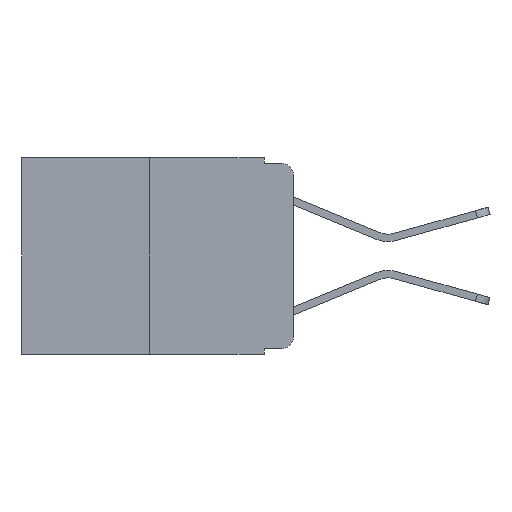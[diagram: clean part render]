
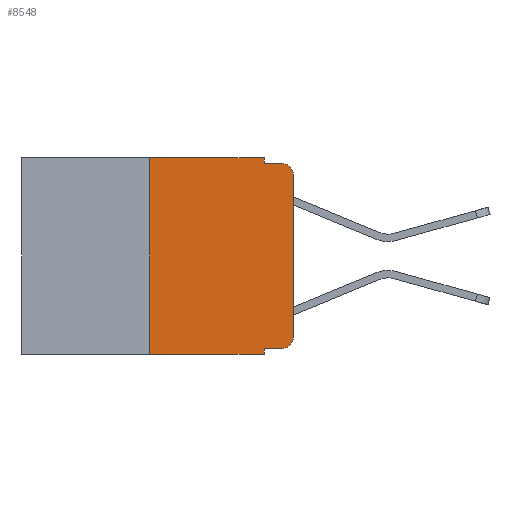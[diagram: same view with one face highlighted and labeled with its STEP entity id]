
A CAD part, left-side view. The second image highlights one B-rep face of the part: STEP entity #8548.
In plain terms, the highlighted planar face has unit normal (-1, 0, 0).
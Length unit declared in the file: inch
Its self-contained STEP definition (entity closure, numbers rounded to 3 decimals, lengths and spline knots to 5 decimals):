
#337 = ORIENTED_EDGE ( 'NONE', *, *, #23741, .T. ) ;
#712 = CARTESIAN_POINT ( 'NONE',  ( 0., 0.051, -0.01 ) ) ;
#1247 = DIRECTION ( 'NONE',  ( 0., 0., -1. ) ) ;
#1405 = LINE ( 'NONE', #23690, #12093 ) ;
#1639 = EDGE_CURVE ( 'NONE', #9684, #12475, #24835, .T. ) ;
#2132 = EDGE_CURVE ( 'NONE', #7017, #9684, #1405, .T. ) ;
#2565 = LINE ( 'NONE', #17969, #22277 ) ;
#2589 = ORIENTED_EDGE ( 'NONE', *, *, #8407, .F. ) ;
#3540 = LINE ( 'NONE', #712, #12911 ) ;
#3730 = DIRECTION ( 'NONE',  ( 0., 0., 1. ) ) ;
#3855 = ORIENTED_EDGE ( 'NONE', *, *, #16317, .F. ) ;
#4034 = CARTESIAN_POINT ( 'NONE',  ( 0., 0.051, 0. ) ) ;
#4226 = VECTOR ( 'NONE', #25190, 39.37008 ) ;
#4394 = CARTESIAN_POINT ( 'NONE',  ( 0., 0.02, -0.01 ) ) ;
#4492 = ORIENTED_EDGE ( 'NONE', *, *, #23707, .T. ) ;
#4607 = VECTOR ( 'NONE', #18806, 39.37008 ) ;
#5143 = ORIENTED_EDGE ( 'NONE', *, *, #25364, .T. ) ;
#5808 = CARTESIAN_POINT ( 'NONE',  ( 0., 0.473, -0.343 ) ) ;
#6491 = CARTESIAN_POINT ( 'NONE',  ( 0., 0., -0.313 ) ) ;
#6852 = DIRECTION ( 'NONE',  ( 0., -1., 0. ) ) ;
#7017 = VERTEX_POINT ( 'NONE', #6491 ) ;
#7067 = CARTESIAN_POINT ( 'NONE',  ( 0., 0.25, 0. ) ) ;
#7165 = CIRCLE ( 'NONE', #21109, 0.02 ) ;
#7187 = EDGE_LOOP ( 'NONE', ( #11993, #17793, #2589, #18398, #13854, #3855, #4492, #15078, #5143, #337 ) ) ;
#7448 = CARTESIAN_POINT ( 'NONE',  ( 0., 0.051, -0.333 ) ) ;
#7570 = CARTESIAN_POINT ( 'NONE',  ( 0., 0.02, -0.333 ) ) ;
#7597 = VERTEX_POINT ( 'NONE', #12286 ) ;
#7981 = DIRECTION ( 'NONE',  ( -1., 0., 0. ) ) ;
#8093 = DIRECTION ( 'NONE',  ( 0., 0., -1. ) ) ;
#8407 = EDGE_CURVE ( 'NONE', #10711, #12475, #3540, .T. ) ;
#8548 = ADVANCED_FACE ( 'NONE', ( #24096 ), #20976, .F. ) ;
#8761 = VERTEX_POINT ( 'NONE', #10605 ) ;
#9382 = AXIS2_PLACEMENT_3D ( 'NONE', #22905, #13267, #1247 ) ;
#9659 = VERTEX_POINT ( 'NONE', #7570 ) ;
#9683 = VECTOR ( 'NONE', #10834, 39.37008 ) ;
#9684 = VERTEX_POINT ( 'NONE', #23248 ) ;
#10303 = LINE ( 'NONE', #24439, #9683 ) ;
#10605 = CARTESIAN_POINT ( 'NONE',  ( 0., 0.051, 0. ) ) ;
#10711 = VERTEX_POINT ( 'NONE', #20444 ) ;
#10834 = DIRECTION ( 'NONE',  ( 0., -1., 0. ) ) ;
#11993 = ORIENTED_EDGE ( 'NONE', *, *, #2132, .T. ) ;
#12093 = VECTOR ( 'NONE', #3730, 39.37008 ) ;
#12286 = CARTESIAN_POINT ( 'NONE',  ( 0., 0.25, 0. ) ) ;
#12402 = EDGE_CURVE ( 'NONE', #8761, #10711, #2565, .T. ) ;
#12475 = VERTEX_POINT ( 'NONE', #4394 ) ;
#12911 = VECTOR ( 'NONE', #6852, 39.37008 ) ;
#13267 = DIRECTION ( 'NONE',  ( 1., 0., 0. ) ) ;
#13854 = ORIENTED_EDGE ( 'NONE', *, *, #20328, .F. ) ;
#14845 = VECTOR ( 'NONE', #23573, 39.37008 ) ;
#15078 = ORIENTED_EDGE ( 'NONE', *, *, #22115, .F. ) ;
#15691 = CARTESIAN_POINT ( 'NONE',  ( 0., 0.25, -0.343 ) ) ;
#16317 = EDGE_CURVE ( 'NONE', #16575, #7597, #20311, .T. ) ;
#16575 = VERTEX_POINT ( 'NONE', #15691 ) ;
#17610 = VECTOR ( 'NONE', #19607, 39.37008 ) ;
#17793 = ORIENTED_EDGE ( 'NONE', *, *, #1639, .T. ) ;
#17969 = CARTESIAN_POINT ( 'NONE',  ( 0., 0.051, 0. ) ) ;
#18398 = ORIENTED_EDGE ( 'NONE', *, *, #12402, .F. ) ;
#18806 = DIRECTION ( 'NONE',  ( 0., 0., 1. ) ) ;
#19282 = CARTESIAN_POINT ( 'NONE',  ( 0., 0.02, -0.03 ) ) ;
#19555 = VERTEX_POINT ( 'NONE', #22244 ) ;
#19607 = DIRECTION ( 'NONE',  ( 0., -1., 0. ) ) ;
#19686 = CARTESIAN_POINT ( 'NONE',  ( 0., 0.02, -0.313 ) ) ;
#19774 = AXIS2_PLACEMENT_3D ( 'NONE', #19282, #24227, #24234 ) ;
#19926 = LINE ( 'NONE', #21319, #4226 ) ;
#20311 = LINE ( 'NONE', #7067, #4607 ) ;
#20328 = EDGE_CURVE ( 'NONE', #7597, #8761, #10303, .T. ) ;
#20444 = CARTESIAN_POINT ( 'NONE',  ( 0., 0.051, -0.01 ) ) ;
#20976 = PLANE ( 'NONE',  #9382 ) ;
#21109 = AXIS2_PLACEMENT_3D ( 'NONE', #19686, #7981, #21631 ) ;
#21110 = VERTEX_POINT ( 'NONE', #7448 ) ;
#21319 = CARTESIAN_POINT ( 'NONE',  ( 0., 0.051, -0.333 ) ) ;
#21631 = DIRECTION ( 'NONE',  ( 0., 0., -1. ) ) ;
#22115 = EDGE_CURVE ( 'NONE', #21110, #19555, #24501, .T. ) ;
#22244 = CARTESIAN_POINT ( 'NONE',  ( 0., 0.051, -0.343 ) ) ;
#22277 = VECTOR ( 'NONE', #8093, 39.37008 ) ;
#22733 = LINE ( 'NONE', #5808, #17610 ) ;
#22905 = CARTESIAN_POINT ( 'NONE',  ( 0., 0.473, 0. ) ) ;
#23248 = CARTESIAN_POINT ( 'NONE',  ( 0., 0., -0.03 ) ) ;
#23573 = DIRECTION ( 'NONE',  ( 0., 0., -1. ) ) ;
#23690 = CARTESIAN_POINT ( 'NONE',  ( 0., 0., 0. ) ) ;
#23707 = EDGE_CURVE ( 'NONE', #16575, #19555, #22733, .T. ) ;
#23741 = EDGE_CURVE ( 'NONE', #9659, #7017, #7165, .T. ) ;
#24096 = FACE_OUTER_BOUND ( 'NONE', #7187, .T. ) ;
#24227 = DIRECTION ( 'NONE',  ( -1., 0., 0. ) ) ;
#24234 = DIRECTION ( 'NONE',  ( 0., 0., -1. ) ) ;
#24439 = CARTESIAN_POINT ( 'NONE',  ( 0., 0.473, 0. ) ) ;
#24501 = LINE ( 'NONE', #4034, #14845 ) ;
#24835 = CIRCLE ( 'NONE', #19774, 0.02 ) ;
#25190 = DIRECTION ( 'NONE',  ( 0., -1., 0. ) ) ;
#25364 = EDGE_CURVE ( 'NONE', #21110, #9659, #19926, .T. ) ;
